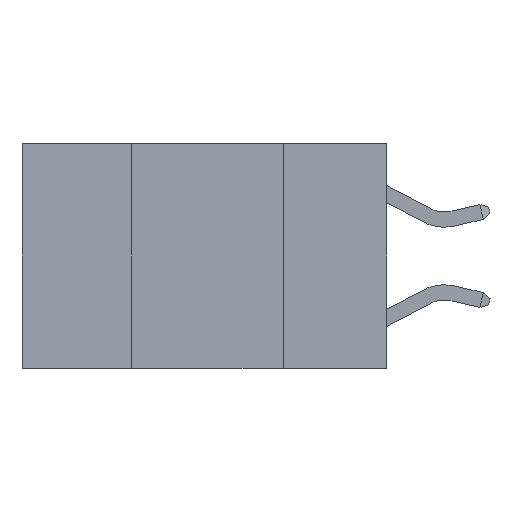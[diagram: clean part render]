
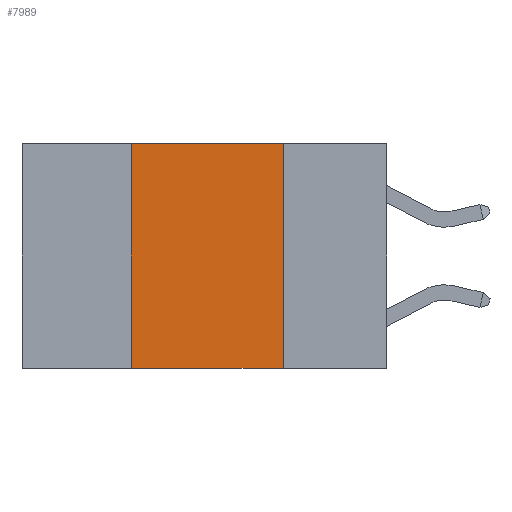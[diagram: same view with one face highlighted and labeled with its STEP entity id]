
A CAD part, left-side view. The second image highlights one B-rep face of the part: STEP entity #7989.
In plain terms, the highlighted planar face has unit normal (-1, 0, 0).
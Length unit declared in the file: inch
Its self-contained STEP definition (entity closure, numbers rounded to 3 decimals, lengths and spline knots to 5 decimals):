
#188 = EDGE_LOOP ( 'NONE', ( #19525, #13019, #17324, #12855 ) ) ;
#3623 = VECTOR ( 'NONE', #12419, 39.37008 ) ;
#4965 = DIRECTION ( 'NONE',  ( 0., 0., -1. ) ) ;
#5069 = VECTOR ( 'NONE', #6338, 39.37008 ) ;
#5952 = VECTOR ( 'NONE', #14342, 39.37008 ) ;
#6338 = DIRECTION ( 'NONE',  ( 0., -1., 0. ) ) ;
#6618 = LINE ( 'NONE', #12316, #5952 ) ;
#7738 = EDGE_CURVE ( 'NONE', #25752, #21062, #6618, .T. ) ;
#7989 = ADVANCED_FACE ( 'NONE', ( #10455 ), #15135, .F. ) ;
#9752 = LINE ( 'NONE', #22395, #3623 ) ;
#10455 = FACE_OUTER_BOUND ( 'NONE', #188, .T. ) ;
#11750 = DIRECTION ( 'NONE',  ( 0., -1., 0. ) ) ;
#12124 = VERTEX_POINT ( 'NONE', #17781 ) ;
#12316 = CARTESIAN_POINT ( 'NONE',  ( 0., 0.42, 0. ) ) ;
#12419 = DIRECTION ( 'NONE',  ( 0., 0., -1. ) ) ;
#12855 = ORIENTED_EDGE ( 'NONE', *, *, #19923, .T. ) ;
#13019 = ORIENTED_EDGE ( 'NONE', *, *, #23303, .F. ) ;
#14342 = DIRECTION ( 'NONE',  ( 0., 0., 1. ) ) ;
#15133 = VECTOR ( 'NONE', #11750, 39.37008 ) ;
#15135 = PLANE ( 'NONE',  #17592 ) ;
#15892 = LINE ( 'NONE', #16461, #5069 ) ;
#16411 = VERTEX_POINT ( 'NONE', #17839 ) ;
#16461 = CARTESIAN_POINT ( 'NONE',  ( 0., 0.6, -0.37 ) ) ;
#16797 = CARTESIAN_POINT ( 'NONE',  ( 0., 0.42, 0. ) ) ;
#17171 = DIRECTION ( 'NONE',  ( 1., 0., 0. ) ) ;
#17324 = ORIENTED_EDGE ( 'NONE', *, *, #7738, .F. ) ;
#17592 = AXIS2_PLACEMENT_3D ( 'NONE', #23083, #17171, #4965 ) ;
#17746 = CARTESIAN_POINT ( 'NONE',  ( 0., 0.6, 0. ) ) ;
#17781 = CARTESIAN_POINT ( 'NONE',  ( 0., 0.17, -0.37 ) ) ;
#17839 = CARTESIAN_POINT ( 'NONE',  ( 0., 0.17, 0. ) ) ;
#19525 = ORIENTED_EDGE ( 'NONE', *, *, #23931, .F. ) ;
#19923 = EDGE_CURVE ( 'NONE', #25752, #12124, #15892, .T. ) ;
#20437 = LINE ( 'NONE', #17746, #15133 ) ;
#21062 = VERTEX_POINT ( 'NONE', #16797 ) ;
#22138 = CARTESIAN_POINT ( 'NONE',  ( 0., 0.42, -0.37 ) ) ;
#22395 = CARTESIAN_POINT ( 'NONE',  ( 0., 0.17, 0. ) ) ;
#23083 = CARTESIAN_POINT ( 'NONE',  ( 0., 0.6, 0. ) ) ;
#23303 = EDGE_CURVE ( 'NONE', #21062, #16411, #20437, .T. ) ;
#23931 = EDGE_CURVE ( 'NONE', #16411, #12124, #9752, .T. ) ;
#25752 = VERTEX_POINT ( 'NONE', #22138 ) ;
